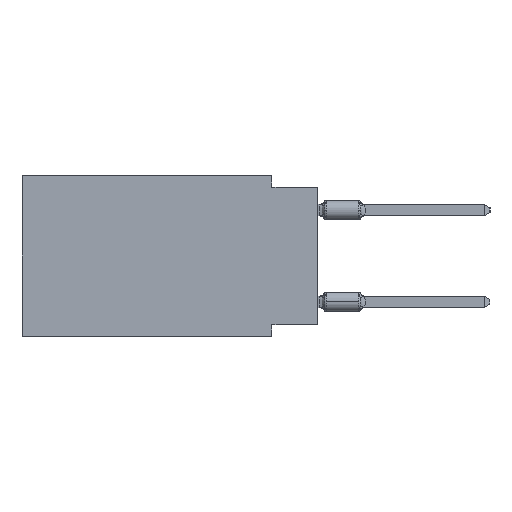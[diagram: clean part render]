
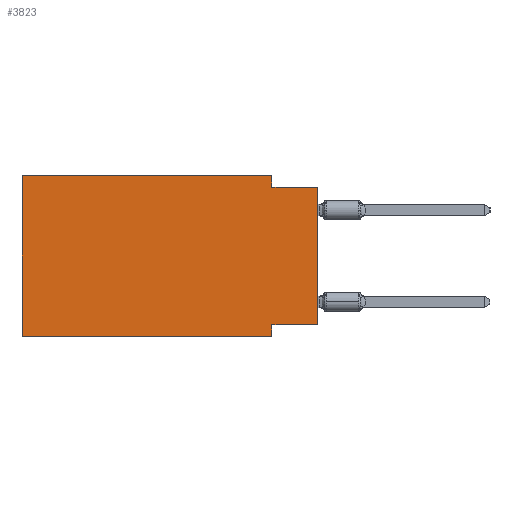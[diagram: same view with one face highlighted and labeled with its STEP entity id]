
A CAD part, left-side view. The second image highlights one B-rep face of the part: STEP entity #3823.
In plain terms, the highlighted planar face has unit normal (-1, 0, 0).
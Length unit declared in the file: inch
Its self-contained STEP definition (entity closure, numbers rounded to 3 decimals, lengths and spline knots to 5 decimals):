
#311 = VECTOR ( 'NONE', #7850, 39.37008 ) ;
#316 = LINE ( 'NONE', #17227, #11374 ) ;
#459 = DIRECTION ( 'NONE',  ( 0., -1., 0. ) ) ;
#511 = ORIENTED_EDGE ( 'NONE', *, *, #13887, .F. ) ;
#780 = DIRECTION ( 'NONE',  ( 0., 0., 1. ) ) ;
#1150 = ORIENTED_EDGE ( 'NONE', *, *, #28472, .T. ) ;
#1427 = EDGE_CURVE ( 'NONE', #20683, #15716, #9109, .T. ) ;
#1509 = DIRECTION ( 'NONE',  ( 0., 1., 0. ) ) ;
#1590 = DIRECTION ( 'NONE',  ( 0., 0., 1. ) ) ;
#2295 = CARTESIAN_POINT ( 'NONE',  ( 0., 0., -0.025 ) ) ;
#3291 = ORIENTED_EDGE ( 'NONE', *, *, #30995, .F. ) ;
#3823 = ADVANCED_FACE ( 'NONE', ( #14908 ), #18070, .F. ) ;
#3949 = DIRECTION ( 'NONE',  ( 0., -1., 0. ) ) ;
#4156 = EDGE_LOOP ( 'NONE', ( #1150, #32717, #11991, #6681, #7799, #36427, #511, #3291 ) ) ;
#5332 = VERTEX_POINT ( 'NONE', #16754 ) ;
#5913 = VERTEX_POINT ( 'NONE', #17649 ) ;
#6681 = ORIENTED_EDGE ( 'NONE', *, *, #24386, .F. ) ;
#7160 = CARTESIAN_POINT ( 'NONE',  ( 0., 0., 0. ) ) ;
#7468 = VECTOR ( 'NONE', #780, 39.37008 ) ;
#7799 = ORIENTED_EDGE ( 'NONE', *, *, #1427, .F. ) ;
#7850 = DIRECTION ( 'NONE',  ( 0., -1., 0. ) ) ;
#8212 = LINE ( 'NONE', #30883, #29681 ) ;
#8278 = CARTESIAN_POINT ( 'NONE',  ( 0., 0.645, 0. ) ) ;
#8796 = CARTESIAN_POINT ( 'NONE',  ( 0., 0., -0.325 ) ) ;
#9109 = LINE ( 'NONE', #26581, #7468 ) ;
#11374 = VECTOR ( 'NONE', #22790, 39.37008 ) ;
#11404 = LINE ( 'NONE', #8278, #29625 ) ;
#11991 = ORIENTED_EDGE ( 'NONE', *, *, #16058, .F. ) ;
#12987 = VERTEX_POINT ( 'NONE', #33642 ) ;
#13887 = EDGE_CURVE ( 'NONE', #5332, #15154, #8212, .T. ) ;
#14908 = FACE_OUTER_BOUND ( 'NONE', #4156, .T. ) ;
#15154 = VERTEX_POINT ( 'NONE', #19543 ) ;
#15716 = VERTEX_POINT ( 'NONE', #23013 ) ;
#16058 = EDGE_CURVE ( 'NONE', #17860, #12987, #316, .T. ) ;
#16517 = VECTOR ( 'NONE', #3949, 39.37008 ) ;
#16754 = CARTESIAN_POINT ( 'NONE',  ( 0., 0.1, -0.325 ) ) ;
#17227 = CARTESIAN_POINT ( 'NONE',  ( 0., 0.1, 0. ) ) ;
#17649 = CARTESIAN_POINT ( 'NONE',  ( 0., 0., -0.025 ) ) ;
#17860 = VERTEX_POINT ( 'NONE', #30110 ) ;
#18070 = PLANE ( 'NONE',  #29184 ) ;
#18271 = DIRECTION ( 'NONE',  ( 1., 0., 0. ) ) ;
#19242 = VECTOR ( 'NONE', #1509, 39.37008 ) ;
#19543 = CARTESIAN_POINT ( 'NONE',  ( 0., 0.1, -0.35 ) ) ;
#20683 = VERTEX_POINT ( 'NONE', #27107 ) ;
#21241 = LINE ( 'NONE', #7160, #35225 ) ;
#21965 = LINE ( 'NONE', #2295, #311 ) ;
#22098 = EDGE_CURVE ( 'NONE', #20683, #15154, #34931, .T. ) ;
#22790 = DIRECTION ( 'NONE',  ( 0., 0., -1. ) ) ;
#23013 = CARTESIAN_POINT ( 'NONE',  ( 0., 0.645, 0. ) ) ;
#23833 = CARTESIAN_POINT ( 'NONE',  ( 0., 0.645, 0. ) ) ;
#24386 = EDGE_CURVE ( 'NONE', #15716, #17860, #11404, .T. ) ;
#25297 = DIRECTION ( 'NONE',  ( 0., 0., -1. ) ) ;
#26581 = CARTESIAN_POINT ( 'NONE',  ( 0., 0.645, 0. ) ) ;
#27031 = VERTEX_POINT ( 'NONE', #8796 ) ;
#27107 = CARTESIAN_POINT ( 'NONE',  ( 0., 0.645, -0.35 ) ) ;
#28472 = EDGE_CURVE ( 'NONE', #27031, #5913, #21241, .T. ) ;
#29184 = AXIS2_PLACEMENT_3D ( 'NONE', #23833, #18271, #29788 ) ;
#29366 = CARTESIAN_POINT ( 'NONE',  ( 0., 0.645, -0.35 ) ) ;
#29445 = EDGE_CURVE ( 'NONE', #12987, #5913, #21965, .T. ) ;
#29625 = VECTOR ( 'NONE', #459, 39.37008 ) ;
#29681 = VECTOR ( 'NONE', #25297, 39.37008 ) ;
#29788 = DIRECTION ( 'NONE',  ( 0., 0., -1. ) ) ;
#30110 = CARTESIAN_POINT ( 'NONE',  ( 0., 0.1, 0. ) ) ;
#30883 = CARTESIAN_POINT ( 'NONE',  ( 0., 0.1, -0.35 ) ) ;
#30995 = EDGE_CURVE ( 'NONE', #27031, #5332, #32310, .T. ) ;
#32310 = LINE ( 'NONE', #35456, #19242 ) ;
#32717 = ORIENTED_EDGE ( 'NONE', *, *, #29445, .F. ) ;
#33642 = CARTESIAN_POINT ( 'NONE',  ( 0., 0.1, -0.025 ) ) ;
#34931 = LINE ( 'NONE', #29366, #16517 ) ;
#35225 = VECTOR ( 'NONE', #1590, 39.37008 ) ;
#35456 = CARTESIAN_POINT ( 'NONE',  ( 0., 0., -0.325 ) ) ;
#36427 = ORIENTED_EDGE ( 'NONE', *, *, #22098, .T. ) ;
